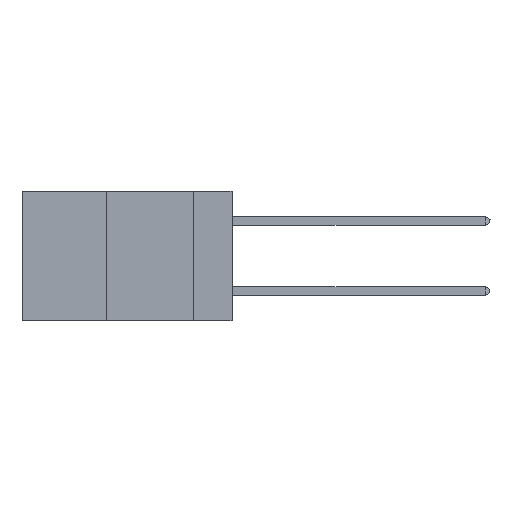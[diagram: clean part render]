
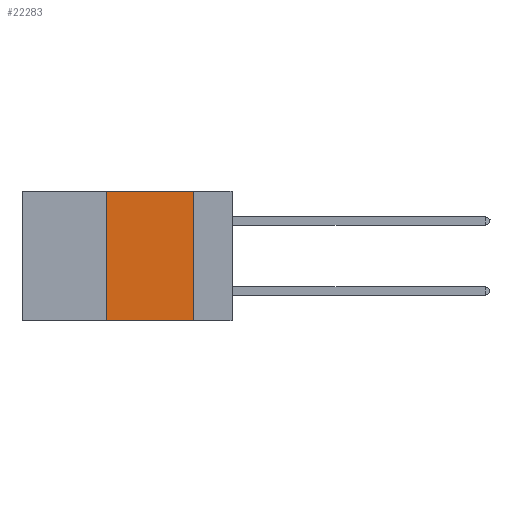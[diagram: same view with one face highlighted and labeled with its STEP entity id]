
A CAD part, left-side view. The second image highlights one B-rep face of the part: STEP entity #22283.
In plain terms, the highlighted planar face has unit normal (-1, 0, 0).
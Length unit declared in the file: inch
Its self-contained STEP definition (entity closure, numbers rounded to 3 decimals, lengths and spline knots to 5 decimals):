
#3317 = CARTESIAN_POINT ( 'NONE',  ( 0., 0.11, 0. ) ) ;
#3939 = VERTEX_POINT ( 'NONE', #33314 ) ;
#5009 = PLANE ( 'NONE',  #10203 ) ;
#6710 = VERTEX_POINT ( 'NONE', #3317 ) ;
#6730 = LINE ( 'NONE', #13588, #23684 ) ;
#7479 = LINE ( 'NONE', #29971, #33571 ) ;
#7712 = CARTESIAN_POINT ( 'NONE',  ( 0., 0.6, 0. ) ) ;
#8244 = ORIENTED_EDGE ( 'NONE', *, *, #46075, .T. ) ;
#10141 = VERTEX_POINT ( 'NONE', #36430 ) ;
#10175 = ORIENTED_EDGE ( 'NONE', *, *, #37832, .F. ) ;
#10203 = AXIS2_PLACEMENT_3D ( 'NONE', #45851, #46092, #46576 ) ;
#10294 = ORIENTED_EDGE ( 'NONE', *, *, #13904, .F. ) ;
#11145 = DIRECTION ( 'NONE',  ( 0., 0., 1. ) ) ;
#11809 = EDGE_LOOP ( 'NONE', ( #10294, #10175, #22188, #8244 ) ) ;
#13588 = CARTESIAN_POINT ( 'NONE',  ( 0., 0.6, -0.37 ) ) ;
#13904 = EDGE_CURVE ( 'NONE', #6710, #3939, #25639, .T. ) ;
#15851 = EDGE_CURVE ( 'NONE', #10141, #27311, #7479, .T. ) ;
#22188 = ORIENTED_EDGE ( 'NONE', *, *, #15851, .F. ) ;
#22283 = ADVANCED_FACE ( 'NONE', ( #31169 ), #5009, .F. ) ;
#23684 = VECTOR ( 'NONE', #28495, 39.37008 ) ;
#25639 = LINE ( 'NONE', #36131, #36535 ) ;
#27311 = VERTEX_POINT ( 'NONE', #40191 ) ;
#28495 = DIRECTION ( 'NONE',  ( 0., -1., 0. ) ) ;
#28816 = DIRECTION ( 'NONE',  ( 0., 0., -1. ) ) ;
#29965 = DIRECTION ( 'NONE',  ( 0., -1., 0. ) ) ;
#29971 = CARTESIAN_POINT ( 'NONE',  ( 0., 0.36, 0. ) ) ;
#31169 = FACE_OUTER_BOUND ( 'NONE', #11809, .T. ) ;
#31452 = VECTOR ( 'NONE', #29965, 39.37008 ) ;
#33314 = CARTESIAN_POINT ( 'NONE',  ( 0., 0.11, -0.37 ) ) ;
#33571 = VECTOR ( 'NONE', #11145, 39.37008 ) ;
#36131 = CARTESIAN_POINT ( 'NONE',  ( 0., 0.11, 0. ) ) ;
#36430 = CARTESIAN_POINT ( 'NONE',  ( 0., 0.36, -0.37 ) ) ;
#36535 = VECTOR ( 'NONE', #28816, 39.37008 ) ;
#37832 = EDGE_CURVE ( 'NONE', #27311, #6710, #37997, .T. ) ;
#37997 = LINE ( 'NONE', #7712, #31452 ) ;
#40191 = CARTESIAN_POINT ( 'NONE',  ( 0., 0.36, 0. ) ) ;
#45851 = CARTESIAN_POINT ( 'NONE',  ( 0., 0.6, 0. ) ) ;
#46075 = EDGE_CURVE ( 'NONE', #10141, #3939, #6730, .T. ) ;
#46092 = DIRECTION ( 'NONE',  ( 1., 0., 0. ) ) ;
#46576 = DIRECTION ( 'NONE',  ( 0., 0., -1. ) ) ;
